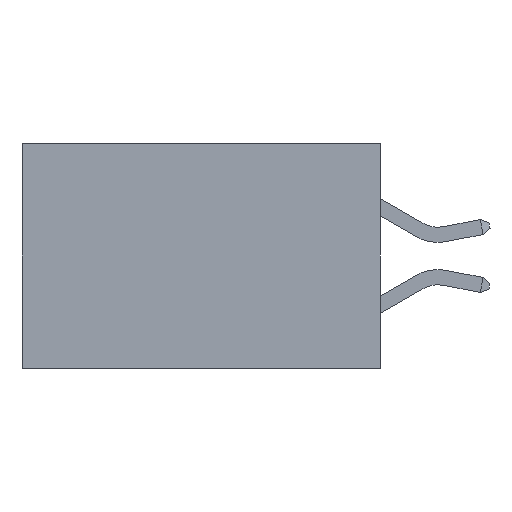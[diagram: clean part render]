
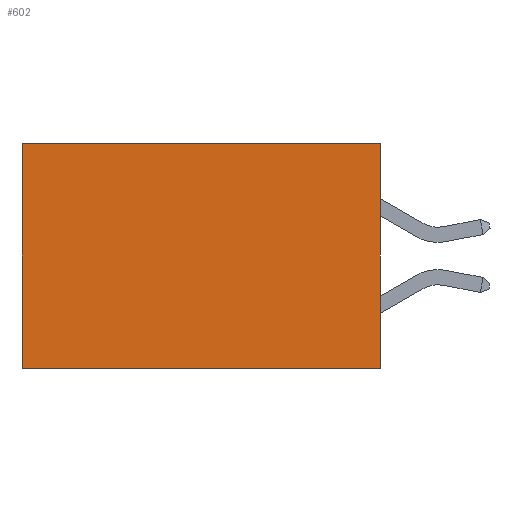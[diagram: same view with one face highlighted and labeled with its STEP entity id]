
A CAD part, left-side view. The second image highlights one B-rep face of the part: STEP entity #602.
In plain terms, the highlighted planar face has unit normal (-1, 0, 0).
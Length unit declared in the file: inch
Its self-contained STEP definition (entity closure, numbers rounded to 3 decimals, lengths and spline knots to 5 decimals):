
#22 = CARTESIAN_POINT ( 'NONE',  ( 0.277, 0., 0. ) ) ;
#123 = DIRECTION ( 'NONE',  ( 0., 1., 0. ) ) ;
#136 = DIRECTION ( 'NONE',  ( 0., 1., 0. ) ) ;
#397 = CARTESIAN_POINT ( 'NONE',  ( 0.277, 0.59, 0. ) ) ;
#419 = CARTESIAN_POINT ( 'NONE',  ( 0.277, 0., 0. ) ) ;
#602 = ADVANCED_FACE ( 'NONE', ( #6711 ), #6883, .F. ) ;
#846 = VECTOR ( 'NONE', #6442, 39.37008 ) ;
#863 = DIRECTION ( 'NONE',  ( 0., 0., -1. ) ) ;
#1089 = LINE ( 'NONE', #6275, #846 ) ;
#1266 = CARTESIAN_POINT ( 'NONE',  ( 0.277, 0., -0.37 ) ) ;
#1302 = EDGE_CURVE ( 'NONE', #6382, #3587, #4249, .T. ) ;
#1629 = AXIS2_PLACEMENT_3D ( 'NONE', #5226, #2833, #5716 ) ;
#2830 = EDGE_LOOP ( 'NONE', ( #5304, #6954, #8690, #3754 ) ) ;
#2833 = DIRECTION ( 'NONE',  ( 1., 0., 0. ) ) ;
#3587 = VERTEX_POINT ( 'NONE', #8616 ) ;
#3720 = CARTESIAN_POINT ( 'NONE',  ( 0.277, 0.59, -0.37 ) ) ;
#3754 = ORIENTED_EDGE ( 'NONE', *, *, #5362, .T. ) ;
#3866 = VECTOR ( 'NONE', #123, 39.37008 ) ;
#4249 = LINE ( 'NONE', #3720, #7499 ) ;
#5226 = CARTESIAN_POINT ( 'NONE',  ( 0.277, 0., -0.37 ) ) ;
#5304 = ORIENTED_EDGE ( 'NONE', *, *, #1302, .T. ) ;
#5349 = EDGE_CURVE ( 'NONE', #8279, #3587, #5829, .T. ) ;
#5362 = EDGE_CURVE ( 'NONE', #6369, #6382, #7274, .T. ) ;
#5621 = VECTOR ( 'NONE', #136, 39.37008 ) ;
#5716 = DIRECTION ( 'NONE',  ( 0., 0., -1. ) ) ;
#5829 = LINE ( 'NONE', #1266, #3866 ) ;
#6250 = CARTESIAN_POINT ( 'NONE',  ( 0.277, 0., -0.37 ) ) ;
#6275 = CARTESIAN_POINT ( 'NONE',  ( 0.277, 0., -0.37 ) ) ;
#6369 = VERTEX_POINT ( 'NONE', #419 ) ;
#6382 = VERTEX_POINT ( 'NONE', #397 ) ;
#6442 = DIRECTION ( 'NONE',  ( 0., 0., -1. ) ) ;
#6711 = FACE_OUTER_BOUND ( 'NONE', #2830, .T. ) ;
#6883 = PLANE ( 'NONE',  #1629 ) ;
#6954 = ORIENTED_EDGE ( 'NONE', *, *, #5349, .F. ) ;
#7022 = EDGE_CURVE ( 'NONE', #6369, #8279, #1089, .T. ) ;
#7274 = LINE ( 'NONE', #22, #5621 ) ;
#7499 = VECTOR ( 'NONE', #863, 39.37008 ) ;
#8279 = VERTEX_POINT ( 'NONE', #6250 ) ;
#8616 = CARTESIAN_POINT ( 'NONE',  ( 0.277, 0.59, -0.37 ) ) ;
#8690 = ORIENTED_EDGE ( 'NONE', *, *, #7022, .F. ) ;
